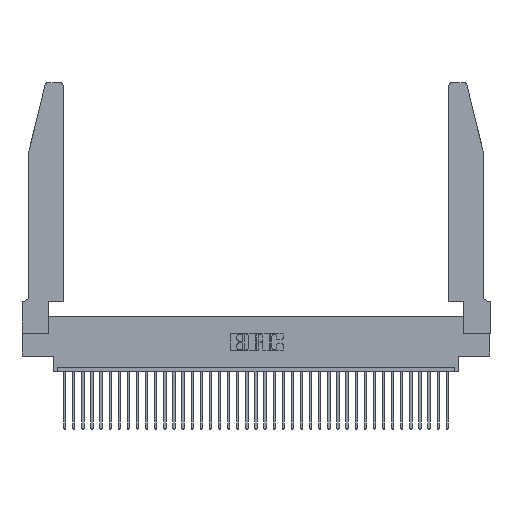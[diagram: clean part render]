
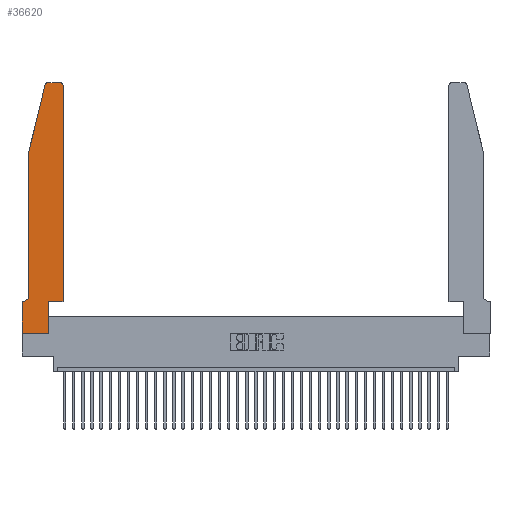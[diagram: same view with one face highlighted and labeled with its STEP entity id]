
A CAD part, top view. The second image highlights one B-rep face of the part: STEP entity #36620.
In plain terms, the highlighted planar face has unit normal (0, 0, 1).
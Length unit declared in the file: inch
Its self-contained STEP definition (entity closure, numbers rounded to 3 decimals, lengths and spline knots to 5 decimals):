
#59 = DIRECTION ( 'NONE',  ( 1., 0., 0. ) ) ;
#358 = AXIS2_PLACEMENT_3D ( 'NONE', #7282, #16255, #30301 ) ;
#438 = CARTESIAN_POINT ( 'NONE',  ( 0.4205, 2.75, 0.37 ) ) ;
#1154 = ORIENTED_EDGE ( 'NONE', *, *, #3072, .T. ) ;
#2287 = EDGE_CURVE ( 'NONE', #2998, #36431, #17552, .T. ) ;
#2318 = VECTOR ( 'NONE', #59, 39.37008 ) ;
#2420 = DIRECTION ( 'NONE',  ( -1., 0., 0. ) ) ;
#2996 = VERTEX_POINT ( 'NONE', #34037 ) ;
#2998 = VERTEX_POINT ( 'NONE', #34166 ) ;
#3072 = EDGE_CURVE ( 'NONE', #7896, #34363, #26349, .T. ) ;
#3600 = FACE_OUTER_BOUND ( 'NONE', #19265, .T. ) ;
#3637 = ORIENTED_EDGE ( 'NONE', *, *, #23090, .T. ) ;
#4469 = AXIS2_PLACEMENT_3D ( 'NONE', #28024, #11218, #22416 ) ;
#4585 = ORIENTED_EDGE ( 'NONE', *, *, #20459, .T. ) ;
#4809 = VECTOR ( 'NONE', #22689, 39.37008 ) ;
#5163 = LINE ( 'NONE', #29613, #9159 ) ;
#5470 = EDGE_CURVE ( 'NONE', #2996, #14157, #15111, .T. ) ;
#5950 = LINE ( 'NONE', #21165, #31019 ) ;
#6702 = CARTESIAN_POINT ( 'NONE',  ( 0.284, 2.75, 0.37 ) ) ;
#6933 = DIRECTION ( 'NONE',  ( 1., 0., 0. ) ) ;
#6942 = ORIENTED_EDGE ( 'NONE', *, *, #24832, .T. ) ;
#7282 = CARTESIAN_POINT ( 'NONE',  ( 0., 0.35, 0.37 ) ) ;
#7416 = PLANE ( 'NONE',  #358 ) ;
#7873 = VERTEX_POINT ( 'NONE', #13758 ) ;
#7896 = VERTEX_POINT ( 'NONE', #27900 ) ;
#8372 = ORIENTED_EDGE ( 'NONE', *, *, #16330, .T. ) ;
#8668 = LINE ( 'NONE', #31041, #28758 ) ;
#8851 = LINE ( 'NONE', #23215, #19167 ) ;
#9159 = VECTOR ( 'NONE', #15434, 39.37008 ) ;
#9762 = VERTEX_POINT ( 'NONE', #16919 ) ;
#9929 = DIRECTION ( 'NONE',  ( 1., 0., 0. ) ) ;
#11166 = DIRECTION ( 'NONE',  ( 0., 1., 0. ) ) ;
#11218 = DIRECTION ( 'NONE',  ( 0., 0., -1. ) ) ;
#11335 = CARTESIAN_POINT ( 'NONE',  ( 0.0755, 2., 0.37 ) ) ;
#12125 = DIRECTION ( 'NONE',  ( 0., 0., 1. ) ) ;
#12163 = CARTESIAN_POINT ( 'NONE',  ( 0.0055, 0.35, 0.37 ) ) ;
#12477 = ORIENTED_EDGE ( 'NONE', *, *, #31800, .T. ) ;
#12759 = CARTESIAN_POINT ( 'NONE',  ( 0.4505, 2.72, 0.37 ) ) ;
#12970 = EDGE_CURVE ( 'NONE', #34363, #2996, #28983, .T. ) ;
#13758 = CARTESIAN_POINT ( 'NONE',  ( 0.2865, 0., 0.37 ) ) ;
#13907 = CARTESIAN_POINT ( 'NONE',  ( 0.0755, 0.35, 0.37 ) ) ;
#14157 = VERTEX_POINT ( 'NONE', #12163 ) ;
#14423 = EDGE_CURVE ( 'NONE', #21393, #9762, #26239, .T. ) ;
#15111 = CIRCLE ( 'NONE', #4469, 0.07 ) ;
#15169 = ORIENTED_EDGE ( 'NONE', *, *, #27598, .T. ) ;
#15246 = CIRCLE ( 'NONE', #23513, 0.03 ) ;
#15434 = DIRECTION ( 'NONE',  ( -1., 0., 0. ) ) ;
#16255 = DIRECTION ( 'NONE',  ( 0., 0., 1. ) ) ;
#16330 = EDGE_CURVE ( 'NONE', #14157, #21393, #35536, .T. ) ;
#16645 = VECTOR ( 'NONE', #19886, 39.37008 ) ;
#16919 = CARTESIAN_POINT ( 'NONE',  ( 0., 0., 0.37 ) ) ;
#17552 = LINE ( 'NONE', #30147, #2318 ) ;
#17719 = ORIENTED_EDGE ( 'NONE', *, *, #5470, .T. ) ;
#17799 = CIRCLE ( 'NONE', #20537, 0.03 ) ;
#18366 = DIRECTION ( 'NONE',  ( 0., 0., 1. ) ) ;
#18568 = DIRECTION ( 'NONE',  ( 0., -1., 0. ) ) ;
#18766 = ORIENTED_EDGE ( 'NONE', *, *, #18972, .T. ) ;
#18972 = EDGE_CURVE ( 'NONE', #29088, #30014, #5163, .T. ) ;
#19167 = VECTOR ( 'NONE', #11166, 39.37008 ) ;
#19265 = EDGE_LOOP ( 'NONE', ( #18766, #6942, #1154, #23443, #17719, #8372, #27552, #4585, #3637, #21677, #15169, #12477 ) ) ;
#19886 = DIRECTION ( 'NONE',  ( -0.239, -0.971, 0. ) ) ;
#20459 = EDGE_CURVE ( 'NONE', #9762, #7873, #5950, .T. ) ;
#20537 = AXIS2_PLACEMENT_3D ( 'NONE', #32477, #18366, #6933 ) ;
#21165 = CARTESIAN_POINT ( 'NONE',  ( 0., 0., 0.37 ) ) ;
#21393 = VERTEX_POINT ( 'NONE', #28360 ) ;
#21427 = VECTOR ( 'NONE', #18568, 39.37008 ) ;
#21677 = ORIENTED_EDGE ( 'NONE', *, *, #2287, .T. ) ;
#21930 = CARTESIAN_POINT ( 'NONE',  ( 0.0755, 2., 0.37 ) ) ;
#22416 = DIRECTION ( 'NONE',  ( -1., 0., 0. ) ) ;
#22689 = DIRECTION ( 'NONE',  ( 0., -1., 0. ) ) ;
#22692 = VERTEX_POINT ( 'NONE', #12759 ) ;
#23090 = EDGE_CURVE ( 'NONE', #7873, #2998, #8851, .T. ) ;
#23215 = CARTESIAN_POINT ( 'NONE',  ( 0.2865, 0.35, 0.37 ) ) ;
#23443 = ORIENTED_EDGE ( 'NONE', *, *, #12970, .T. ) ;
#23513 = AXIS2_PLACEMENT_3D ( 'NONE', #23553, #12125, #32083 ) ;
#23553 = CARTESIAN_POINT ( 'NONE',  ( 0.4205, 2.72, 0.37 ) ) ;
#23795 = CARTESIAN_POINT ( 'NONE',  ( 0.4505, 0.35, 0.37 ) ) ;
#24832 = EDGE_CURVE ( 'NONE', #30014, #7896, #17799, .T. ) ;
#26239 = LINE ( 'NONE', #34200, #4809 ) ;
#26349 = LINE ( 'NONE', #11335, #16645 ) ;
#26559 = VECTOR ( 'NONE', #2420, 39.37008 ) ;
#27552 = ORIENTED_EDGE ( 'NONE', *, *, #14423, .T. ) ;
#27598 = EDGE_CURVE ( 'NONE', #36431, #22692, #8668, .T. ) ;
#27900 = CARTESIAN_POINT ( 'NONE',  ( 0.25487, 2.72718, 0.37 ) ) ;
#28024 = CARTESIAN_POINT ( 'NONE',  ( 0.0055, 0.42, 0.37 ) ) ;
#28360 = CARTESIAN_POINT ( 'NONE',  ( 0., 0.35, 0.37 ) ) ;
#28758 = VECTOR ( 'NONE', #37017, 39.37008 ) ;
#28983 = LINE ( 'NONE', #34701, #21427 ) ;
#29088 = VERTEX_POINT ( 'NONE', #438 ) ;
#29613 = CARTESIAN_POINT ( 'NONE',  ( 0.2605, 2.75, 0.37 ) ) ;
#30014 = VERTEX_POINT ( 'NONE', #6702 ) ;
#30147 = CARTESIAN_POINT ( 'NONE',  ( 0.4505, 0.35, 0.37 ) ) ;
#30301 = DIRECTION ( 'NONE',  ( 1., 0., 0. ) ) ;
#31019 = VECTOR ( 'NONE', #9929, 39.37008 ) ;
#31041 = CARTESIAN_POINT ( 'NONE',  ( 0.4505, 0.35, 0.37 ) ) ;
#31800 = EDGE_CURVE ( 'NONE', #22692, #29088, #15246, .T. ) ;
#32083 = DIRECTION ( 'NONE',  ( 1., 0., 0. ) ) ;
#32477 = CARTESIAN_POINT ( 'NONE',  ( 0.284, 2.72, 0.37 ) ) ;
#34037 = CARTESIAN_POINT ( 'NONE',  ( 0.0755, 0.42, 0.37 ) ) ;
#34166 = CARTESIAN_POINT ( 'NONE',  ( 0.2865, 0.35, 0.37 ) ) ;
#34200 = CARTESIAN_POINT ( 'NONE',  ( 0., 0., 0.37 ) ) ;
#34363 = VERTEX_POINT ( 'NONE', #21930 ) ;
#34701 = CARTESIAN_POINT ( 'NONE',  ( 0.0755, 2., 0.37 ) ) ;
#35536 = LINE ( 'NONE', #13907, #26559 ) ;
#36431 = VERTEX_POINT ( 'NONE', #23795 ) ;
#36620 = ADVANCED_FACE ( 'NONE', ( #3600 ), #7416, .T. ) ;
#37017 = DIRECTION ( 'NONE',  ( 0., 1., 0. ) ) ;
